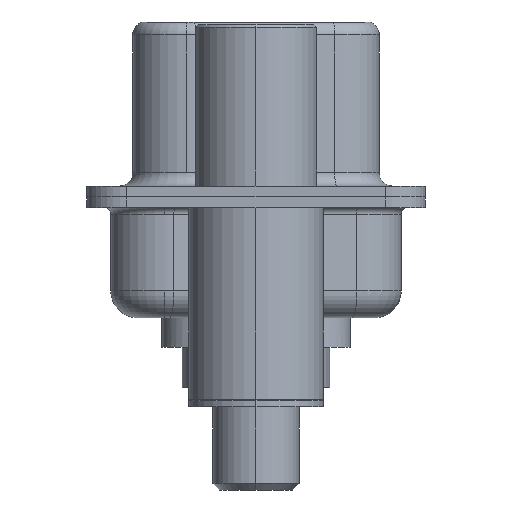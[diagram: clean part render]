
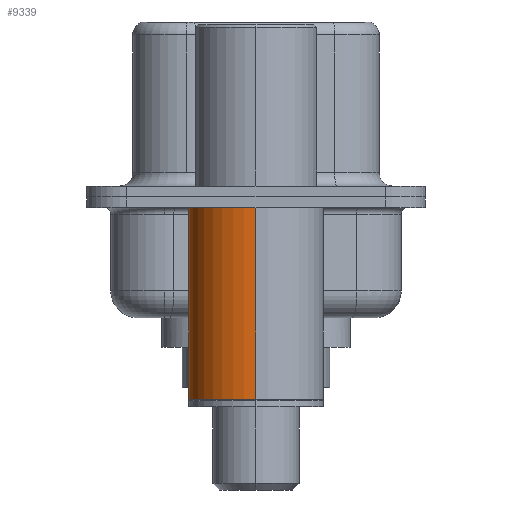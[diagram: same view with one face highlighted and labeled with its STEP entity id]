
A CAD part, left-side view. The second image highlights one B-rep face of the part: STEP entity #9339.
In plain terms, the highlighted cylindrical face has radius 2.5 mm (diameter 5 mm), a partial arc.
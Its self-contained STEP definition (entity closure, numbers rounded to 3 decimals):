
#291 = CIRCLE ( 'NONE', #7404, 2.5 ) ;
#384 = ORIENTED_EDGE ( 'NONE', *, *, #3932, .F. ) ;
#508 = VERTEX_POINT ( 'NONE', #1164 ) ;
#618 = CARTESIAN_POINT ( 'NONE',  ( -2.5, 0., -0.4 ) ) ;
#1062 = DIRECTION ( 'NONE',  ( 1., 0., 0. ) ) ;
#1164 = CARTESIAN_POINT ( 'NONE',  ( 2.5, 0., -7.525 ) ) ;
#1276 = CARTESIAN_POINT ( 'NONE',  ( 2.5, 0., -0.4 ) ) ;
#1296 = EDGE_LOOP ( 'NONE', ( #8376, #9750, #384, #14978 ) ) ;
#1394 = DIRECTION ( 'NONE',  ( 0., 0., 1. ) ) ;
#2737 = CARTESIAN_POINT ( 'NONE',  ( -2.5, 0., 0.581 ) ) ;
#3192 = CARTESIAN_POINT ( 'NONE',  ( 0., 0., -0.4 ) ) ;
#3687 = VERTEX_POINT ( 'NONE', #1276 ) ;
#3932 = EDGE_CURVE ( 'NONE', #3687, #6944, #18145, .T. ) ;
#4771 = DIRECTION ( 'NONE',  ( 0., 0., 1. ) ) ;
#5430 = DIRECTION ( 'NONE',  ( 1., 0., 0. ) ) ;
#5822 = CARTESIAN_POINT ( 'NONE',  ( 2.5, 0., 0.581 ) ) ;
#5991 = FACE_OUTER_BOUND ( 'NONE', #1296, .T. ) ;
#6944 = VERTEX_POINT ( 'NONE', #618 ) ;
#7404 = AXIS2_PLACEMENT_3D ( 'NONE', #14470, #4771, #16062 ) ;
#8376 = ORIENTED_EDGE ( 'NONE', *, *, #19696, .T. ) ;
#9339 = ADVANCED_FACE ( 'NONE', ( #5991 ), #17842, .T. ) ;
#9750 = ORIENTED_EDGE ( 'NONE', *, *, #11163, .T. ) ;
#11163 = EDGE_CURVE ( 'NONE', #19449, #6944, #19831, .T. ) ;
#11238 = VECTOR ( 'NONE', #12531, 1000. ) ;
#12531 = DIRECTION ( 'NONE',  ( 0., 0., 1. ) ) ;
#12865 = CARTESIAN_POINT ( 'NONE',  ( -2.5, 0., -7.525 ) ) ;
#13666 = LINE ( 'NONE', #5822, #21279 ) ;
#13869 = AXIS2_PLACEMENT_3D ( 'NONE', #21104, #14635, #5430 ) ;
#14379 = EDGE_CURVE ( 'NONE', #508, #3687, #13666, .T. ) ;
#14470 = CARTESIAN_POINT ( 'NONE',  ( 0., 0., -7.525 ) ) ;
#14635 = DIRECTION ( 'NONE',  ( 0., 0., 1. ) ) ;
#14978 = ORIENTED_EDGE ( 'NONE', *, *, #14379, .F. ) ;
#15452 = DIRECTION ( 'NONE',  ( 0., 0., 1. ) ) ;
#16062 = DIRECTION ( 'NONE',  ( 1., 0., 0. ) ) ;
#17842 = CYLINDRICAL_SURFACE ( 'NONE', #13869, 2.5 ) ;
#18145 = CIRCLE ( 'NONE', #19787, 2.5 ) ;
#19449 = VERTEX_POINT ( 'NONE', #12865 ) ;
#19696 = EDGE_CURVE ( 'NONE', #508, #19449, #291, .T. ) ;
#19787 = AXIS2_PLACEMENT_3D ( 'NONE', #3192, #1394, #1062 ) ;
#19831 = LINE ( 'NONE', #2737, #11238 ) ;
#21104 = CARTESIAN_POINT ( 'NONE',  ( 0., 0., 0.581 ) ) ;
#21279 = VECTOR ( 'NONE', #15452, 1000. ) ;
